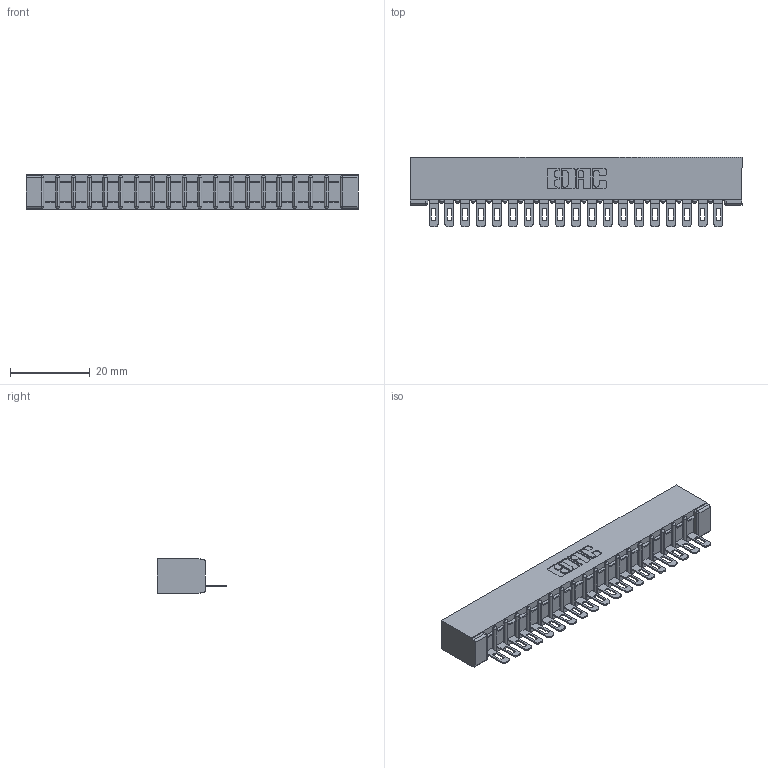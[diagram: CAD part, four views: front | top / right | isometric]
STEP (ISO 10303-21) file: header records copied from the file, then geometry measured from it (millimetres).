
FILE_DESCRIPTION (( 'STEP AP203' ), '1' );
FILE_NAME ('307-019-401-101.STEP', '2020-09-27T00:39:05', ( '' ), ( '' ), 'SwSTEP 2.0', 'SolidWorks 2020', '' );
FILE_SCHEMA (( 'CONFIG_CONTROL_DESIGN' ));
Length unit declared in the file: inch
Products named in the file (3): 307 Part_No Mounting Lugs; 307-290-002_501; 307-019-401-101
Assembly tree (20 placements, depth 2):
  307-019-401-101
    307 Part_No Mounting Lugs
    307-290-002_501  x19
Bounding box: 83.16 x 17.42 x 8.71 mm (x, y, z)
Volume: 5747.3 mm3; surface area: 10921.7 mm2
Topology: 20 solids, 20 shells, 1574 faces, 4821 edges, 3158 vertices
Faces by surface type: plane 902, cylinder 632, sphere 40
Entity records: 19640 total; most frequent: CARTESIAN_POINT 3308, ORIENTED_EDGE 3298, DIRECTION 3227, EDGE_CURVE 1649, LINE 1249, VECTOR 1249, VERTEX_POINT 1070, AXIS2_PLACEMENT_3D 989
